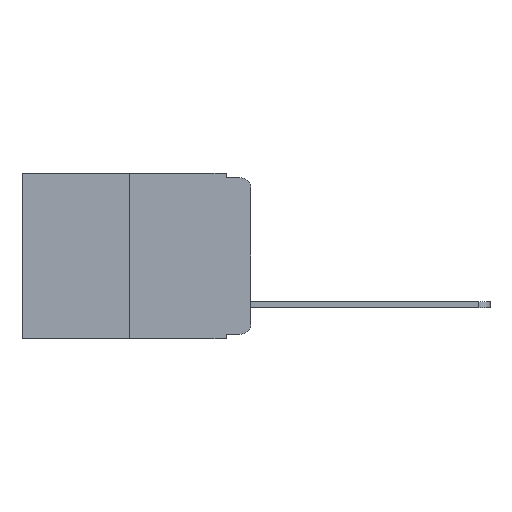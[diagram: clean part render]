
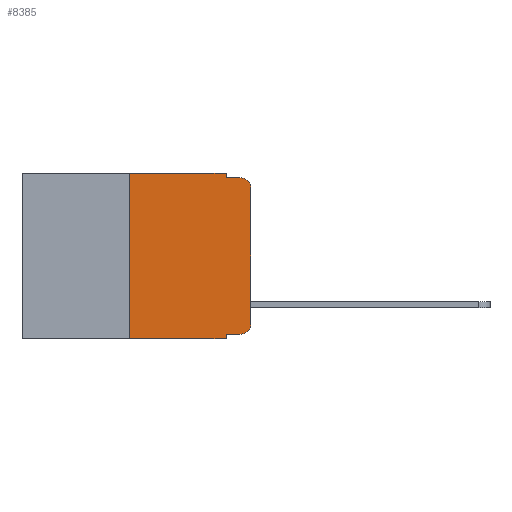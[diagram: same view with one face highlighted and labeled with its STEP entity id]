
A CAD part, left-side view. The second image highlights one B-rep face of the part: STEP entity #8385.
In plain terms, the highlighted planar face has unit normal (-1, 0, 0).
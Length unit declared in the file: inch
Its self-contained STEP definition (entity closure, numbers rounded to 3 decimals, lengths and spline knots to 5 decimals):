
#168 = VERTEX_POINT ( 'NONE', #4251 ) ;
#427 = AXIS2_PLACEMENT_3D ( 'NONE', #7123, #5962, #11308 ) ;
#618 = ORIENTED_EDGE ( 'NONE', *, *, #12724, .T. ) ;
#742 = VERTEX_POINT ( 'NONE', #15529 ) ;
#1160 = EDGE_CURVE ( 'NONE', #9897, #1684, #6622, .T. ) ;
#1257 = PLANE ( 'NONE',  #14682 ) ;
#1587 = DIRECTION ( 'NONE',  ( 0., 0., 1. ) ) ;
#1684 = VERTEX_POINT ( 'NONE', #16708 ) ;
#1717 = VERTEX_POINT ( 'NONE', #2908 ) ;
#1786 = CARTESIAN_POINT ( 'NONE',  ( 0., 0.051, -0.01 ) ) ;
#2089 = CARTESIAN_POINT ( 'NONE',  ( 0., 0.473, 0. ) ) ;
#2253 = CARTESIAN_POINT ( 'NONE',  ( 0., 0.02, -0.01 ) ) ;
#2675 = LINE ( 'NONE', #9811, #13950 ) ;
#2908 = CARTESIAN_POINT ( 'NONE',  ( 0., 0.25, -0.343 ) ) ;
#2917 = ORIENTED_EDGE ( 'NONE', *, *, #6959, .F. ) ;
#2954 = EDGE_CURVE ( 'NONE', #8609, #12632, #16964, .T. ) ;
#3772 = LINE ( 'NONE', #10226, #11214 ) ;
#3965 = CARTESIAN_POINT ( 'NONE',  ( 0., 0.051, -0.333 ) ) ;
#4251 = CARTESIAN_POINT ( 'NONE',  ( 0., 0.25, 0. ) ) ;
#4331 = ORIENTED_EDGE ( 'NONE', *, *, #17073, .T. ) ;
#4476 = VECTOR ( 'NONE', #8717, 39.37008 ) ;
#5335 = DIRECTION ( 'NONE',  ( 1., 0., 0. ) ) ;
#5380 = CIRCLE ( 'NONE', #427, 0.02 ) ;
#5813 = ORIENTED_EDGE ( 'NONE', *, *, #11212, .F. ) ;
#5962 = DIRECTION ( 'NONE',  ( -1., 0., 0. ) ) ;
#6146 = LINE ( 'NONE', #12060, #12953 ) ;
#6340 = ORIENTED_EDGE ( 'NONE', *, *, #17507, .T. ) ;
#6517 = DIRECTION ( 'NONE',  ( 0., 0., -1. ) ) ;
#6622 = LINE ( 'NONE', #11297, #4476 ) ;
#6959 = EDGE_CURVE ( 'NONE', #742, #8609, #6146, .T. ) ;
#7123 = CARTESIAN_POINT ( 'NONE',  ( 0., 0.02, -0.03 ) ) ;
#7369 = DIRECTION ( 'NONE',  ( 0., 0., 1. ) ) ;
#7576 = CIRCLE ( 'NONE', #9844, 0.02 ) ;
#8109 = CARTESIAN_POINT ( 'NONE',  ( 0., 0., -0.313 ) ) ;
#8178 = ORIENTED_EDGE ( 'NONE', *, *, #2954, .F. ) ;
#8330 = FACE_OUTER_BOUND ( 'NONE', #8437, .T. ) ;
#8385 = ADVANCED_FACE ( 'NONE', ( #8330 ), #1257, .F. ) ;
#8437 = EDGE_LOOP ( 'NONE', ( #618, #6340, #8178, #2917, #12919, #5813, #4331, #14764, #15073, #11863 ) ) ;
#8454 = DIRECTION ( 'NONE',  ( 0., -1., 0. ) ) ;
#8601 = LINE ( 'NONE', #12409, #12207 ) ;
#8609 = VERTEX_POINT ( 'NONE', #13317 ) ;
#8694 = VECTOR ( 'NONE', #8703, 39.37008 ) ;
#8703 = DIRECTION ( 'NONE',  ( 0., -1., 0. ) ) ;
#8717 = DIRECTION ( 'NONE',  ( 0., 0., -1. ) ) ;
#9397 = CARTESIAN_POINT ( 'NONE',  ( 0., 0.02, -0.313 ) ) ;
#9811 = CARTESIAN_POINT ( 'NONE',  ( 0., 0., 0. ) ) ;
#9844 = AXIS2_PLACEMENT_3D ( 'NONE', #9397, #12048, #6517 ) ;
#9897 = VERTEX_POINT ( 'NONE', #13241 ) ;
#10226 = CARTESIAN_POINT ( 'NONE',  ( 0., 0.25, 0. ) ) ;
#10986 = CARTESIAN_POINT ( 'NONE',  ( 0., 0.473, 0. ) ) ;
#11128 = LINE ( 'NONE', #3965, #17532 ) ;
#11171 = LINE ( 'NONE', #2089, #14577 ) ;
#11212 = EDGE_CURVE ( 'NONE', #1717, #168, #3772, .T. ) ;
#11214 = VECTOR ( 'NONE', #7369, 39.37008 ) ;
#11297 = CARTESIAN_POINT ( 'NONE',  ( 0., 0.051, 0. ) ) ;
#11308 = DIRECTION ( 'NONE',  ( 0., 0., -1. ) ) ;
#11863 = ORIENTED_EDGE ( 'NONE', *, *, #13119, .T. ) ;
#12048 = DIRECTION ( 'NONE',  ( -1., 0., 0. ) ) ;
#12060 = CARTESIAN_POINT ( 'NONE',  ( 0., 0.051, 0. ) ) ;
#12207 = VECTOR ( 'NONE', #15302, 39.37008 ) ;
#12242 = DIRECTION ( 'NONE',  ( 0., -1., 0. ) ) ;
#12409 = CARTESIAN_POINT ( 'NONE',  ( 0., 0.473, -0.343 ) ) ;
#12482 = CARTESIAN_POINT ( 'NONE',  ( 0., 0.02, -0.333 ) ) ;
#12540 = VERTEX_POINT ( 'NONE', #12482 ) ;
#12550 = EDGE_CURVE ( 'NONE', #168, #742, #11171, .T. ) ;
#12632 = VERTEX_POINT ( 'NONE', #2253 ) ;
#12724 = EDGE_CURVE ( 'NONE', #15635, #13125, #2675, .T. ) ;
#12919 = ORIENTED_EDGE ( 'NONE', *, *, #12550, .F. ) ;
#12953 = VECTOR ( 'NONE', #13186, 39.37008 ) ;
#13119 = EDGE_CURVE ( 'NONE', #12540, #15635, #7576, .T. ) ;
#13125 = VERTEX_POINT ( 'NONE', #14830 ) ;
#13186 = DIRECTION ( 'NONE',  ( 0., 0., -1. ) ) ;
#13241 = CARTESIAN_POINT ( 'NONE',  ( 0., 0.051, -0.333 ) ) ;
#13317 = CARTESIAN_POINT ( 'NONE',  ( 0., 0.051, -0.01 ) ) ;
#13950 = VECTOR ( 'NONE', #1587, 39.37008 ) ;
#14360 = EDGE_CURVE ( 'NONE', #9897, #12540, #11128, .T. ) ;
#14577 = VECTOR ( 'NONE', #8454, 39.37008 ) ;
#14682 = AXIS2_PLACEMENT_3D ( 'NONE', #10986, #5335, #16367 ) ;
#14764 = ORIENTED_EDGE ( 'NONE', *, *, #1160, .F. ) ;
#14830 = CARTESIAN_POINT ( 'NONE',  ( 0., 0., -0.03 ) ) ;
#15073 = ORIENTED_EDGE ( 'NONE', *, *, #14360, .T. ) ;
#15302 = DIRECTION ( 'NONE',  ( 0., -1., 0. ) ) ;
#15529 = CARTESIAN_POINT ( 'NONE',  ( 0., 0.051, 0. ) ) ;
#15635 = VERTEX_POINT ( 'NONE', #8109 ) ;
#16367 = DIRECTION ( 'NONE',  ( 0., 0., -1. ) ) ;
#16708 = CARTESIAN_POINT ( 'NONE',  ( 0., 0.051, -0.343 ) ) ;
#16964 = LINE ( 'NONE', #1786, #8694 ) ;
#17073 = EDGE_CURVE ( 'NONE', #1717, #1684, #8601, .T. ) ;
#17507 = EDGE_CURVE ( 'NONE', #13125, #12632, #5380, .T. ) ;
#17532 = VECTOR ( 'NONE', #12242, 39.37008 ) ;
